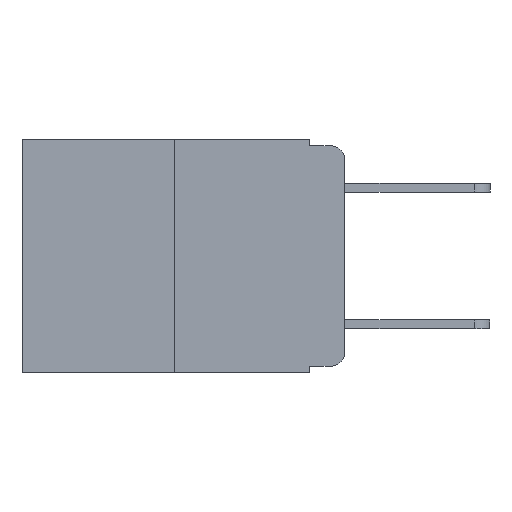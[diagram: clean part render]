
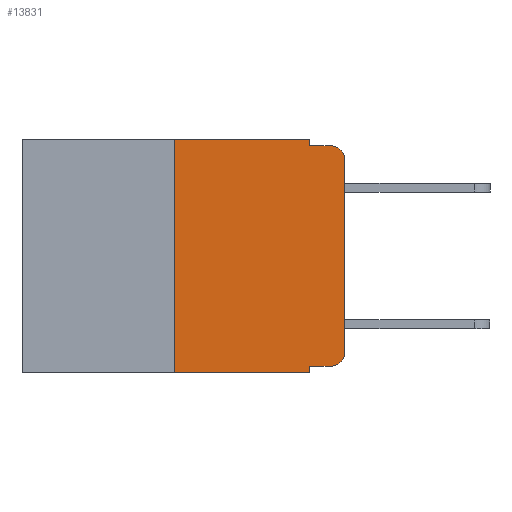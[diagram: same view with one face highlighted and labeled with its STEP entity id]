
A CAD part, left-side view. The second image highlights one B-rep face of the part: STEP entity #13831.
In plain terms, the highlighted planar face has unit normal (-1, 0, 0).
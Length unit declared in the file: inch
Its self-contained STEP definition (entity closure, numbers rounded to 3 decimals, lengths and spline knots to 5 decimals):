
#182 = VECTOR ( 'NONE', #11146, 39.37008 ) ;
#224 = ORIENTED_EDGE ( 'NONE', *, *, #14299, .F. ) ;
#278 = AXIS2_PLACEMENT_3D ( 'NONE', #8219, #16609, #9485 ) ;
#357 = CIRCLE ( 'NONE', #278, 0.02 ) ;
#382 = CARTESIAN_POINT ( 'NONE',  ( 0., 0., 0. ) ) ;
#471 = VERTEX_POINT ( 'NONE', #15151 ) ;
#515 = ORIENTED_EDGE ( 'NONE', *, *, #13213, .T. ) ;
#630 = DIRECTION ( 'NONE',  ( 0., 0., -1. ) ) ;
#1097 = VECTOR ( 'NONE', #12234, 39.37008 ) ;
#1775 = DIRECTION ( 'NONE',  ( 0., 0., -1. ) ) ;
#2115 = VERTEX_POINT ( 'NONE', #9084 ) ;
#2651 = ORIENTED_EDGE ( 'NONE', *, *, #15795, .F. ) ;
#2731 = VECTOR ( 'NONE', #7318, 39.37008 ) ;
#2948 = CARTESIAN_POINT ( 'NONE',  ( 0., 0.051, -0.01 ) ) ;
#2960 = ORIENTED_EDGE ( 'NONE', *, *, #10101, .T. ) ;
#2978 = VERTEX_POINT ( 'NONE', #11655 ) ;
#3177 = ORIENTED_EDGE ( 'NONE', *, *, #12632, .T. ) ;
#3245 = CARTESIAN_POINT ( 'NONE',  ( 0., 0.25, 0. ) ) ;
#3402 = CARTESIAN_POINT ( 'NONE',  ( 0., 0.473, 0. ) ) ;
#3540 = VERTEX_POINT ( 'NONE', #7573 ) ;
#3783 = ORIENTED_EDGE ( 'NONE', *, *, #15028, .T. ) ;
#4396 = CARTESIAN_POINT ( 'NONE',  ( 0., 0.25, 0. ) ) ;
#4918 = EDGE_CURVE ( 'NONE', #12740, #471, #9427, .T. ) ;
#5414 = ORIENTED_EDGE ( 'NONE', *, *, #9057, .F. ) ;
#5477 = ORIENTED_EDGE ( 'NONE', *, *, #6490, .F. ) ;
#6004 = VECTOR ( 'NONE', #12318, 39.37008 ) ;
#6029 = CARTESIAN_POINT ( 'NONE',  ( 0., 0.051, 0. ) ) ;
#6201 = VECTOR ( 'NONE', #12099, 39.37008 ) ;
#6490 = EDGE_CURVE ( 'NONE', #2978, #2115, #11705, .T. ) ;
#6528 = DIRECTION ( 'NONE',  ( -1., 0., 0. ) ) ;
#6681 = ORIENTED_EDGE ( 'NONE', *, *, #4918, .T. ) ;
#7036 = ORIENTED_EDGE ( 'NONE', *, *, #11695, .F. ) ;
#7169 = VERTEX_POINT ( 'NONE', #4396 ) ;
#7318 = DIRECTION ( 'NONE',  ( 0., -1., 0. ) ) ;
#7499 = EDGE_LOOP ( 'NONE', ( #6681, #3783, #5414, #5477, #7036, #224, #515, #2651, #2960, #3177 ) ) ;
#7573 = CARTESIAN_POINT ( 'NONE',  ( 0., 0.051, -0.343 ) ) ;
#7601 = LINE ( 'NONE', #3245, #182 ) ;
#7910 = DIRECTION ( 'NONE',  ( 0., -1., 0. ) ) ;
#8090 = VERTEX_POINT ( 'NONE', #12422 ) ;
#8219 = CARTESIAN_POINT ( 'NONE',  ( 0., 0.02, -0.03 ) ) ;
#8727 = LINE ( 'NONE', #6029, #12363 ) ;
#8848 = DIRECTION ( 'NONE',  ( 1., 0., 0. ) ) ;
#9057 = EDGE_CURVE ( 'NONE', #2115, #9936, #9594, .T. ) ;
#9084 = CARTESIAN_POINT ( 'NONE',  ( 0., 0.051, -0.01 ) ) ;
#9107 = DIRECTION ( 'NONE',  ( 0., -1., 0. ) ) ;
#9427 = LINE ( 'NONE', #382, #6004 ) ;
#9485 = DIRECTION ( 'NONE',  ( 0., 0., -1. ) ) ;
#9594 = LINE ( 'NONE', #2948, #6201 ) ;
#9615 = AXIS2_PLACEMENT_3D ( 'NONE', #3402, #8848, #630 ) ;
#9738 = LINE ( 'NONE', #15189, #12972 ) ;
#9798 = AXIS2_PLACEMENT_3D ( 'NONE', #13929, #6528, #15117 ) ;
#9936 = VERTEX_POINT ( 'NONE', #12425 ) ;
#10093 = CIRCLE ( 'NONE', #9798, 0.02 ) ;
#10101 = EDGE_CURVE ( 'NONE', #12541, #12751, #9738, .T. ) ;
#10313 = VECTOR ( 'NONE', #9107, 39.37008 ) ;
#10534 = CARTESIAN_POINT ( 'NONE',  ( 0., 0., -0.313 ) ) ;
#10592 = CARTESIAN_POINT ( 'NONE',  ( 0., 0.02, -0.333 ) ) ;
#11146 = DIRECTION ( 'NONE',  ( 0., 0., 1. ) ) ;
#11243 = CARTESIAN_POINT ( 'NONE',  ( 0., 0.051, -0.333 ) ) ;
#11655 = CARTESIAN_POINT ( 'NONE',  ( 0., 0.051, 0. ) ) ;
#11695 = EDGE_CURVE ( 'NONE', #7169, #2978, #13150, .T. ) ;
#11705 = LINE ( 'NONE', #13447, #1097 ) ;
#12099 = DIRECTION ( 'NONE',  ( 0., -1., 0. ) ) ;
#12234 = DIRECTION ( 'NONE',  ( 0., 0., -1. ) ) ;
#12318 = DIRECTION ( 'NONE',  ( 0., 0., 1. ) ) ;
#12363 = VECTOR ( 'NONE', #1775, 39.37008 ) ;
#12422 = CARTESIAN_POINT ( 'NONE',  ( 0., 0.25, -0.343 ) ) ;
#12425 = CARTESIAN_POINT ( 'NONE',  ( 0., 0.02, -0.01 ) ) ;
#12541 = VERTEX_POINT ( 'NONE', #11243 ) ;
#12632 = EDGE_CURVE ( 'NONE', #12751, #12740, #10093, .T. ) ;
#12740 = VERTEX_POINT ( 'NONE', #10534 ) ;
#12751 = VERTEX_POINT ( 'NONE', #10592 ) ;
#12972 = VECTOR ( 'NONE', #7910, 39.37008 ) ;
#13150 = LINE ( 'NONE', #16280, #10313 ) ;
#13213 = EDGE_CURVE ( 'NONE', #8090, #3540, #16218, .T. ) ;
#13444 = CARTESIAN_POINT ( 'NONE',  ( 0., 0.473, -0.343 ) ) ;
#13447 = CARTESIAN_POINT ( 'NONE',  ( 0., 0.051, 0. ) ) ;
#13831 = ADVANCED_FACE ( 'NONE', ( #15234 ), #14884, .F. ) ;
#13929 = CARTESIAN_POINT ( 'NONE',  ( 0., 0.02, -0.313 ) ) ;
#14299 = EDGE_CURVE ( 'NONE', #8090, #7169, #7601, .T. ) ;
#14884 = PLANE ( 'NONE',  #9615 ) ;
#15028 = EDGE_CURVE ( 'NONE', #471, #9936, #357, .T. ) ;
#15117 = DIRECTION ( 'NONE',  ( 0., 0., -1. ) ) ;
#15151 = CARTESIAN_POINT ( 'NONE',  ( 0., 0., -0.03 ) ) ;
#15189 = CARTESIAN_POINT ( 'NONE',  ( 0., 0.051, -0.333 ) ) ;
#15234 = FACE_OUTER_BOUND ( 'NONE', #7499, .T. ) ;
#15795 = EDGE_CURVE ( 'NONE', #12541, #3540, #8727, .T. ) ;
#16218 = LINE ( 'NONE', #13444, #2731 ) ;
#16280 = CARTESIAN_POINT ( 'NONE',  ( 0., 0.473, 0. ) ) ;
#16609 = DIRECTION ( 'NONE',  ( -1., 0., 0. ) ) ;
